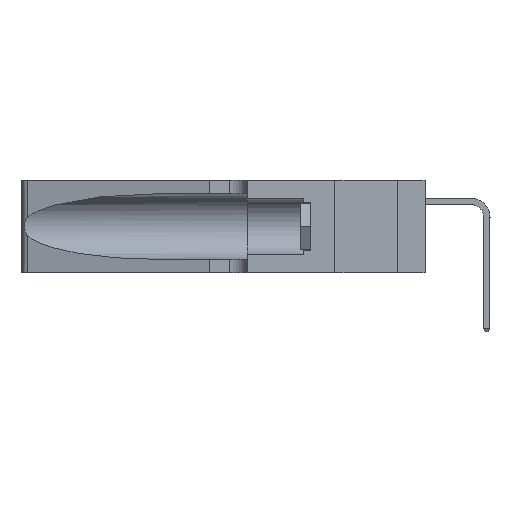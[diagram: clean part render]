
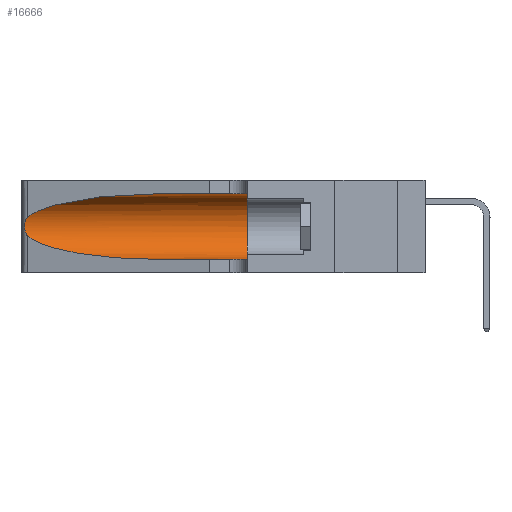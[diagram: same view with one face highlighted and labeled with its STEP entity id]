
A CAD part, left-side view. The second image highlights one B-rep face of the part: STEP entity #16666.
In plain terms, the highlighted cylindrical face has radius 3.308 mm (diameter 6.617 mm), a partial arc.
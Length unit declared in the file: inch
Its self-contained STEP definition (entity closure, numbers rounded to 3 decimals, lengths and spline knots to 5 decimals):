
#933 = CARTESIAN_POINT ( 'NONE',  ( 0.25487, 1.22718, 0.14631 ) ) ;
#1295 = CARTESIAN_POINT ( 'NONE',  ( 0.18966, 0.96281, 0.31525 ) ) ;
#1374 = CARTESIAN_POINT ( 'NONE',  ( 0.25787, 1.23484, 0.2124 ) ) ;
#1730 = ORIENTED_EDGE ( 'NONE', *, *, #29500, .T. ) ;
#2028 = AXIS2_PLACEMENT_3D ( 'NONE', #26384, #16395, #9056 ) ;
#2259 = B_SPLINE_CURVE_WITH_KNOTS ( 'NONE', 3,
 ( #11226, #21064, #16195, #1374, #18651, #3855, #21173, #6350, #23673, #8843, #26176, #11332, #28687, #13808 ),
 .UNSPECIFIED., .F., .F.,
 ( 4, 2, 2, 2, 2, 2, 4 ),
 ( 0., 0.00027, 0.00053, 0.00107, 0.0016, 0.00187, 0.00214 ),
 .UNSPECIFIED. ) ;
#2838 = CARTESIAN_POINT ( 'NONE',  ( 0.25487, 1.22718, 0.14631 ) ) ;
#2989 = ORIENTED_EDGE ( 'NONE', *, *, #29721, .T. ) ;
#3484 = CARTESIAN_POINT ( 'NONE',  ( 0.1305, 0.72297, 0.31525 ) ) ;
#3855 = CARTESIAN_POINT ( 'NONE',  ( 0.26018, 1.23835, 0.19895 ) ) ;
#4105 = AXIS2_PLACEMENT_3D ( 'NONE', #9954, #27286, #12426 ) ;
#6288 = CARTESIAN_POINT ( 'NONE',  ( 0.25487, 1.22718, 0.22369 ) ) ;
#6350 = CARTESIAN_POINT ( 'NONE',  ( 0.26075, 1.23896, 0.178 ) ) ;
#6567 = LINE ( 'NONE', #29093, #12350 ) ;
#6793 = EDGE_CURVE ( 'NONE', #25424, #10316, #22696, .T. ) ;
#7827 = CARTESIAN_POINT ( 'NONE',  ( 0.18966, 0.96281, 0.05475 ) ) ;
#8843 = CARTESIAN_POINT ( 'NONE',  ( 0.25856, 1.23593, 0.16098 ) ) ;
#9056 = DIRECTION ( 'NONE',  ( 0., 0., -1. ) ) ;
#9689 = EDGE_CURVE ( 'NONE', #24155, #25424, #28556, .T. ) ;
#9954 = CARTESIAN_POINT ( 'NONE',  ( 0.1305, 0.35, 0.185 ) ) ;
#10316 = VERTEX_POINT ( 'NONE', #16297 ) ;
#11226 = CARTESIAN_POINT ( 'NONE',  ( 0.25487, 1.22718, 0.22369 ) ) ;
#11332 = CARTESIAN_POINT ( 'NONE',  ( 0.25639, 1.23186, 0.15144 ) ) ;
#12350 = VECTOR ( 'NONE', #16702, 39.37008 ) ;
#12398 = CARTESIAN_POINT ( 'NONE',  ( 0.1305, 0.72297, 0.05475 ) ) ;
#12426 = DIRECTION ( 'NONE',  ( 0., 0., 1. ) ) ;
#13746 =( BOUNDED_CURVE ( )  B_SPLINE_CURVE ( 3, ( #31009, #1295, #21101, #6288 ),
 .UNSPECIFIED., .F., .F. ) 
 B_SPLINE_CURVE_WITH_KNOTS ( ( 4, 4 ),
 ( 1.5708, 2.84003 ),
 .UNSPECIFIED. ) 
 CURVE ( )  GEOMETRIC_REPRESENTATION_ITEM ( )  RATIONAL_B_SPLINE_CURVE ( ( 1., 0.87, 0.87, 1. ) ) 
 REPRESENTATION_ITEM ( '' )  );
#13808 = CARTESIAN_POINT ( 'NONE',  ( 0.25487, 1.22718, 0.14631 ) ) ;
#14023 = EDGE_LOOP ( 'NONE', ( #2989, #24327, #1730, #14546, #18869, #23243 ) ) ;
#14546 = ORIENTED_EDGE ( 'NONE', *, *, #23754, .T. ) ;
#16132 = VECTOR ( 'NONE', #16435, 39.37008 ) ;
#16195 = CARTESIAN_POINT ( 'NONE',  ( 0.25639, 1.23184, 0.21858 ) ) ;
#16297 = CARTESIAN_POINT ( 'NONE',  ( 0.1305, 0.35, 0.05475 ) ) ;
#16395 = DIRECTION ( 'NONE',  ( 0., -1., 0. ) ) ;
#16435 = DIRECTION ( 'NONE',  ( 0., -1., 0. ) ) ;
#16666 = ADVANCED_FACE ( 'NONE', ( #30766 ), #17542, .F. ) ;
#16702 = DIRECTION ( 'NONE',  ( 0., -1., 0. ) ) ;
#17542 = CYLINDRICAL_SURFACE ( 'NONE', #2028, 0.13025 ) ;
#18651 = CARTESIAN_POINT ( 'NONE',  ( 0.25854, 1.2359, 0.20912 ) ) ;
#18869 = ORIENTED_EDGE ( 'NONE', *, *, #6793, .F. ) ;
#19483 =( BOUNDED_CURVE ( )  B_SPLINE_CURVE ( 3, ( #2838, #30055, #7827, #25140 ),
 .UNSPECIFIED., .F., .F. ) 
 B_SPLINE_CURVE_WITH_KNOTS ( ( 4, 4 ),
 ( 3.44316, 4.71239 ),
 .UNSPECIFIED. ) 
 CURVE ( )  GEOMETRIC_REPRESENTATION_ITEM ( )  RATIONAL_B_SPLINE_CURVE ( ( 1., 0.87, 0.87, 1. ) ) 
 REPRESENTATION_ITEM ( '' )  );
#20095 = VERTEX_POINT ( 'NONE', #933 ) ;
#21064 = CARTESIAN_POINT ( 'NONE',  ( 0.25555, 1.22994, 0.2215 ) ) ;
#21101 = CARTESIAN_POINT ( 'NONE',  ( 0.2373, 1.15595, 0.28018 ) ) ;
#21173 = CARTESIAN_POINT ( 'NONE',  ( 0.26075, 1.23896, 0.19203 ) ) ;
#21852 = VERTEX_POINT ( 'NONE', #12398 ) ;
#22696 = CIRCLE ( 'NONE', #4105, 0.13025 ) ;
#23243 = ORIENTED_EDGE ( 'NONE', *, *, #9689, .F. ) ;
#23673 = CARTESIAN_POINT ( 'NONE',  ( 0.26017, 1.23833, 0.17102 ) ) ;
#23754 = EDGE_CURVE ( 'NONE', #21852, #10316, #6567, .T. ) ;
#24155 = VERTEX_POINT ( 'NONE', #3484 ) ;
#24327 = ORIENTED_EDGE ( 'NONE', *, *, #30449, .T. ) ;
#25140 = CARTESIAN_POINT ( 'NONE',  ( 0.1305, 0.72297, 0.05475 ) ) ;
#25424 = VERTEX_POINT ( 'NONE', #25598 ) ;
#25598 = CARTESIAN_POINT ( 'NONE',  ( 0.1305, 0.35, 0.31525 ) ) ;
#26142 = CARTESIAN_POINT ( 'NONE',  ( 0.25487, 1.22718, 0.22369 ) ) ;
#26176 = CARTESIAN_POINT ( 'NONE',  ( 0.25789, 1.23486, 0.15765 ) ) ;
#26384 = CARTESIAN_POINT ( 'NONE',  ( 0.1305, 1.61858, 0.185 ) ) ;
#27286 = DIRECTION ( 'NONE',  ( 0., 1., 0. ) ) ;
#28556 = LINE ( 'NONE', #31320, #16132 ) ;
#28687 = CARTESIAN_POINT ( 'NONE',  ( 0.25555, 1.22993, 0.14849 ) ) ;
#29093 = CARTESIAN_POINT ( 'NONE',  ( 0.1305, 1.61858, 0.05475 ) ) ;
#29146 = VERTEX_POINT ( 'NONE', #26142 ) ;
#29500 = EDGE_CURVE ( 'NONE', #20095, #21852, #19483, .T. ) ;
#29721 = EDGE_CURVE ( 'NONE', #24155, #29146, #13746, .T. ) ;
#30055 = CARTESIAN_POINT ( 'NONE',  ( 0.2373, 1.15595, 0.08982 ) ) ;
#30449 = EDGE_CURVE ( 'NONE', #29146, #20095, #2259, .T. ) ;
#30766 = FACE_OUTER_BOUND ( 'NONE', #14023, .T. ) ;
#31009 = CARTESIAN_POINT ( 'NONE',  ( 0.1305, 0.72297, 0.31525 ) ) ;
#31320 = CARTESIAN_POINT ( 'NONE',  ( 0.1305, 1.61858, 0.31525 ) ) ;
